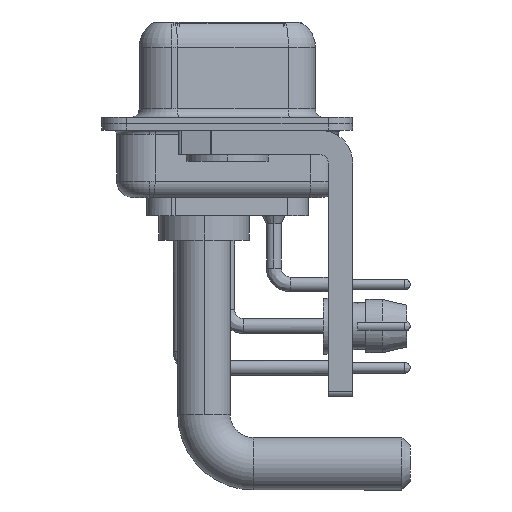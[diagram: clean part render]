
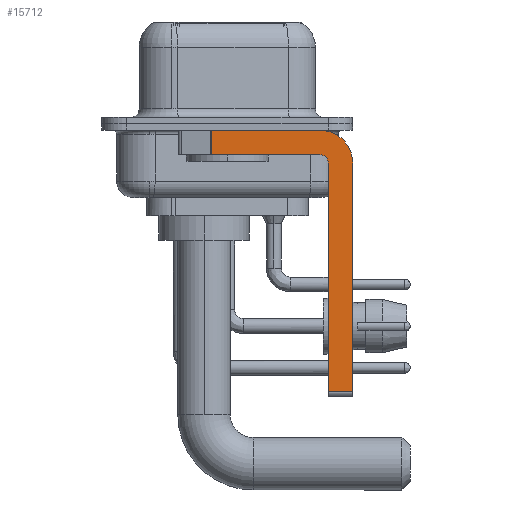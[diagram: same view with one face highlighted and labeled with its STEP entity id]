
A CAD part, left-side view. The second image highlights one B-rep face of the part: STEP entity #15712.
In plain terms, the highlighted planar face has unit normal (-1, 0, 0).
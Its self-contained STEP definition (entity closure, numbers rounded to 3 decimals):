
#176 = EDGE_CURVE ( 'NONE', #7328, #547, #7127, .T. ) ;
#319 = DIRECTION ( 'NONE',  ( 1., 0., 0. ) ) ;
#547 = VERTEX_POINT ( 'NONE', #35942 ) ;
#1800 = EDGE_CURVE ( 'NONE', #34748, #4908, #4166, .T. ) ;
#3087 = VECTOR ( 'NONE', #9149, 1000. ) ;
#4166 = CIRCLE ( 'NONE', #24708, 2. ) ;
#4246 = VERTEX_POINT ( 'NONE', #17491 ) ;
#4417 = VERTEX_POINT ( 'NONE', #24647 ) ;
#4908 = VERTEX_POINT ( 'NONE', #13609 ) ;
#7127 = CIRCLE ( 'NONE', #27689, 0.5 ) ;
#7328 = VERTEX_POINT ( 'NONE', #24586 ) ;
#7848 = DIRECTION ( 'NONE',  ( -1., 0., 0. ) ) ;
#8537 = CARTESIAN_POINT ( 'NONE',  ( -2.9, -7.65, -2.4 ) ) ;
#8769 = VECTOR ( 'NONE', #13130, 1000. ) ;
#8782 = CARTESIAN_POINT ( 'NONE',  ( -2.9, -5.65, -2.4 ) ) ;
#8806 = PLANE ( 'NONE',  #13220 ) ;
#8809 = LINE ( 'NONE', #25884, #3087 ) ;
#8872 = LINE ( 'NONE', #14544, #35253 ) ;
#9149 = DIRECTION ( 'NONE',  ( 0., -1., 0. ) ) ;
#9666 = EDGE_CURVE ( 'NONE', #35634, #34748, #18649, .T. ) ;
#10124 = ORIENTED_EDGE ( 'NONE', *, *, #28859, .T. ) ;
#11442 = LINE ( 'NONE', #8537, #25622 ) ;
#11578 = CARTESIAN_POINT ( 'NONE',  ( -2.9, 0.978, -1.9 ) ) ;
#13130 = DIRECTION ( 'NONE',  ( 0., -1., 0. ) ) ;
#13220 = AXIS2_PLACEMENT_3D ( 'NONE', #19981, #28829, #25708 ) ;
#13229 = ORIENTED_EDGE ( 'NONE', *, *, #34246, .F. ) ;
#13609 = CARTESIAN_POINT ( 'NONE',  ( -2.9, -7.65, -2.4 ) ) ;
#14544 = CARTESIAN_POINT ( 'NONE',  ( -2.9, -5.65, -1.9 ) ) ;
#15712 = ADVANCED_FACE ( 'NONE', ( #33984 ), #8806, .F. ) ;
#16289 = DIRECTION ( 'NONE',  ( 0., 0., 1. ) ) ;
#16478 = EDGE_CURVE ( 'NONE', #4908, #28650, #11442, .T. ) ;
#16953 = DIRECTION ( 'NONE',  ( 0., 1., 0. ) ) ;
#17491 = CARTESIAN_POINT ( 'NONE',  ( -2.9, -6.15, -16.35 ) ) ;
#17968 = EDGE_LOOP ( 'NONE', ( #35760, #10124, #13229, #26368, #29431, #19989, #23190, #21910 ) ) ;
#18649 = LINE ( 'NONE', #19189, #8769 ) ;
#19189 = CARTESIAN_POINT ( 'NONE',  ( -2.9, 3., -0.4 ) ) ;
#19981 = CARTESIAN_POINT ( 'NONE',  ( -2.9, -5.65, -2.4 ) ) ;
#19989 = ORIENTED_EDGE ( 'NONE', *, *, #35555, .T. ) ;
#20709 = CARTESIAN_POINT ( 'NONE',  ( -2.9, 0.978, -0.4 ) ) ;
#21910 = ORIENTED_EDGE ( 'NONE', *, *, #1800, .F. ) ;
#22613 = DIRECTION ( 'NONE',  ( 0., 0., -1. ) ) ;
#23048 = CARTESIAN_POINT ( 'NONE',  ( -2.9, -5.65, -0.4 ) ) ;
#23190 = ORIENTED_EDGE ( 'NONE', *, *, #16478, .F. ) ;
#23343 = LINE ( 'NONE', #11578, #28511 ) ;
#23734 = LINE ( 'NONE', #34615, #24655 ) ;
#24586 = CARTESIAN_POINT ( 'NONE',  ( -2.9, -6.15, -2.4 ) ) ;
#24647 = CARTESIAN_POINT ( 'NONE',  ( -2.9, 0.978, -1.9 ) ) ;
#24655 = VECTOR ( 'NONE', #26136, 1000. ) ;
#24708 = AXIS2_PLACEMENT_3D ( 'NONE', #8782, #319, #33597 ) ;
#25622 = VECTOR ( 'NONE', #33889, 1000. ) ;
#25708 = DIRECTION ( 'NONE',  ( 0., 0., -1. ) ) ;
#25884 = CARTESIAN_POINT ( 'NONE',  ( -2.9, -5.65, -16.35 ) ) ;
#26136 = DIRECTION ( 'NONE',  ( 0., 0., 1. ) ) ;
#26368 = ORIENTED_EDGE ( 'NONE', *, *, #176, .F. ) ;
#27689 = AXIS2_PLACEMENT_3D ( 'NONE', #33025, #7848, #16289 ) ;
#28511 = VECTOR ( 'NONE', #22613, 1000. ) ;
#28650 = VERTEX_POINT ( 'NONE', #32584 ) ;
#28829 = DIRECTION ( 'NONE',  ( 1., 0., 0. ) ) ;
#28859 = EDGE_CURVE ( 'NONE', #35634, #4417, #23343, .T. ) ;
#29431 = ORIENTED_EDGE ( 'NONE', *, *, #34322, .F. ) ;
#32584 = CARTESIAN_POINT ( 'NONE',  ( -2.9, -7.65, -16.35 ) ) ;
#33025 = CARTESIAN_POINT ( 'NONE',  ( -2.9, -5.65, -2.4 ) ) ;
#33597 = DIRECTION ( 'NONE',  ( 0., 0., -1. ) ) ;
#33889 = DIRECTION ( 'NONE',  ( 0., 0., -1. ) ) ;
#33984 = FACE_OUTER_BOUND ( 'NONE', #17968, .T. ) ;
#34246 = EDGE_CURVE ( 'NONE', #547, #4417, #8872, .T. ) ;
#34322 = EDGE_CURVE ( 'NONE', #4246, #7328, #23734, .T. ) ;
#34615 = CARTESIAN_POINT ( 'NONE',  ( -2.9, -6.15, -16.6 ) ) ;
#34748 = VERTEX_POINT ( 'NONE', #23048 ) ;
#35253 = VECTOR ( 'NONE', #16953, 1000. ) ;
#35555 = EDGE_CURVE ( 'NONE', #4246, #28650, #8809, .T. ) ;
#35634 = VERTEX_POINT ( 'NONE', #20709 ) ;
#35760 = ORIENTED_EDGE ( 'NONE', *, *, #9666, .F. ) ;
#35942 = CARTESIAN_POINT ( 'NONE',  ( -2.9, -5.65, -1.9 ) ) ;
